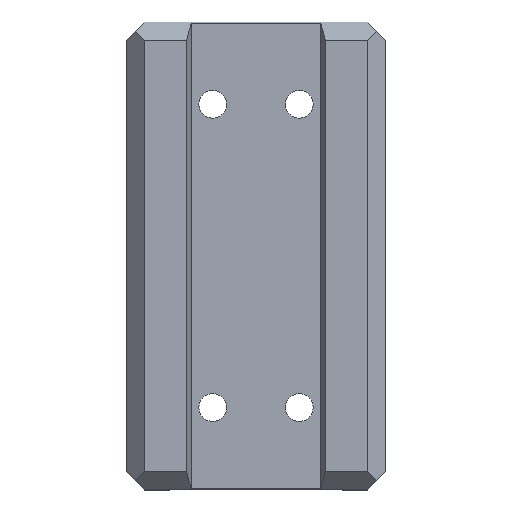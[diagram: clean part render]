
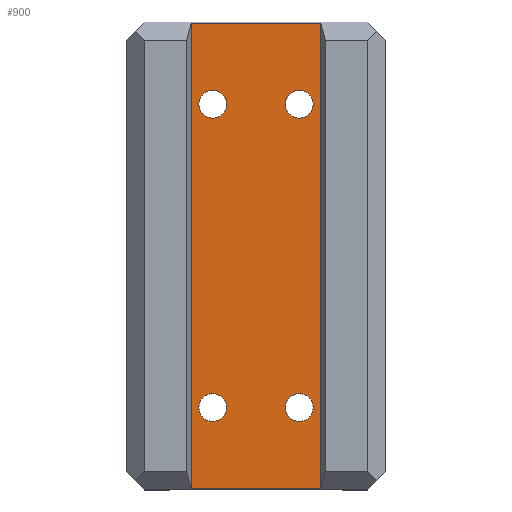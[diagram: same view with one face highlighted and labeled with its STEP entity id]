
A CAD part, top view. The second image highlights one B-rep face of the part: STEP entity #900.
In plain terms, the highlighted planar face has unit normal (0, 0, 1).
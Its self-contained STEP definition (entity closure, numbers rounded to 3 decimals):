
#325 = VERTEX_POINT('',#326);
#326 = CARTESIAN_POINT('',(7.5,-26.884,4.995));
#332 = EDGE_CURVE('',#333,#325,#335,.T.);
#333 = VERTEX_POINT('',#334);
#334 = CARTESIAN_POINT('',(-7.5,-26.884,4.995));
#335 = LINE('',#336,#337);
#336 = CARTESIAN_POINT('',(-7.5,-26.884,4.995));
#337 = VECTOR('',#338,1.);
#338 = DIRECTION('',(1.,0.,-0.));
#414 = VERTEX_POINT('',#415);
#415 = CARTESIAN_POINT('',(-7.5,26.884,4.995));
#421 = EDGE_CURVE('',#422,#414,#424,.T.);
#422 = VERTEX_POINT('',#423);
#423 = CARTESIAN_POINT('',(7.5,26.884,4.995));
#424 = LINE('',#425,#426);
#425 = CARTESIAN_POINT('',(-7.5,26.884,4.995));
#426 = VECTOR('',#427,1.);
#427 = DIRECTION('',(-1.,0.,0.));
#889 = EDGE_CURVE('',#333,#414,#890,.T.);
#890 = LINE('',#891,#892);
#891 = CARTESIAN_POINT('',(-7.5,-27.,4.995));
#892 = VECTOR('',#893,1.);
#893 = DIRECTION('',(0.,1.,0.));
#900 = ADVANCED_FACE('',(#901,#912,#923,#934,#945),#956,.F.);
#901 = FACE_BOUND('',#902,.F.);
#902 = EDGE_LOOP('',(#903,#904,#905,#911));
#903 = ORIENTED_EDGE('',*,*,#889,.T.);
#904 = ORIENTED_EDGE('',*,*,#421,.F.);
#905 = ORIENTED_EDGE('',*,*,#906,.T.);
#906 = EDGE_CURVE('',#422,#325,#907,.T.);
#907 = LINE('',#908,#909);
#908 = CARTESIAN_POINT('',(7.5,27.,4.995));
#909 = VECTOR('',#910,1.);
#910 = DIRECTION('',(0.,-1.,0.));
#911 = ORIENTED_EDGE('',*,*,#332,.F.);
#912 = FACE_BOUND('',#913,.F.);
#913 = EDGE_LOOP('',(#914));
#914 = ORIENTED_EDGE('',*,*,#915,.F.);
#915 = EDGE_CURVE('',#916,#916,#918,.T.);
#916 = VERTEX_POINT('',#917);
#917 = CARTESIAN_POINT('',(6.6,-17.5,4.995));
#918 = CIRCLE('',#919,1.6);
#919 = AXIS2_PLACEMENT_3D('',#920,#921,#922);
#920 = CARTESIAN_POINT('',(5.,-17.5,4.995));
#921 = DIRECTION('',(0.,0.,-1.));
#922 = DIRECTION('',(1.,0.,0.));
#923 = FACE_BOUND('',#924,.F.);
#924 = EDGE_LOOP('',(#925));
#925 = ORIENTED_EDGE('',*,*,#926,.F.);
#926 = EDGE_CURVE('',#927,#927,#929,.T.);
#927 = VERTEX_POINT('',#928);
#928 = CARTESIAN_POINT('',(-3.4,-17.5,4.995));
#929 = CIRCLE('',#930,1.6);
#930 = AXIS2_PLACEMENT_3D('',#931,#932,#933);
#931 = CARTESIAN_POINT('',(-5.,-17.5,4.995));
#932 = DIRECTION('',(0.,0.,-1.));
#933 = DIRECTION('',(1.,0.,0.));
#934 = FACE_BOUND('',#935,.F.);
#935 = EDGE_LOOP('',(#936));
#936 = ORIENTED_EDGE('',*,*,#937,.F.);
#937 = EDGE_CURVE('',#938,#938,#940,.T.);
#938 = VERTEX_POINT('',#939);
#939 = CARTESIAN_POINT('',(6.6,17.5,4.995));
#940 = CIRCLE('',#941,1.6);
#941 = AXIS2_PLACEMENT_3D('',#942,#943,#944);
#942 = CARTESIAN_POINT('',(5.,17.5,4.995));
#943 = DIRECTION('',(0.,0.,-1.));
#944 = DIRECTION('',(1.,0.,0.));
#945 = FACE_BOUND('',#946,.F.);
#946 = EDGE_LOOP('',(#947));
#947 = ORIENTED_EDGE('',*,*,#948,.F.);
#948 = EDGE_CURVE('',#949,#949,#951,.T.);
#949 = VERTEX_POINT('',#950);
#950 = CARTESIAN_POINT('',(-3.4,17.5,4.995));
#951 = CIRCLE('',#952,1.6);
#952 = AXIS2_PLACEMENT_3D('',#953,#954,#955);
#953 = CARTESIAN_POINT('',(-5.,17.5,4.995));
#954 = DIRECTION('',(0.,0.,-1.));
#955 = DIRECTION('',(1.,0.,0.));
#956 = PLANE('',#957);
#957 = AXIS2_PLACEMENT_3D('',#958,#959,#960);
#958 = CARTESIAN_POINT('',(0.,0.,4.995));
#959 = DIRECTION('',(-0.,-0.,-1.));
#960 = DIRECTION('',(-1.,0.,0.));
